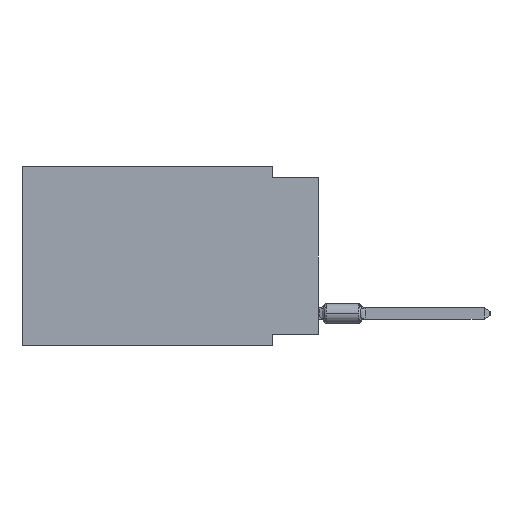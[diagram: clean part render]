
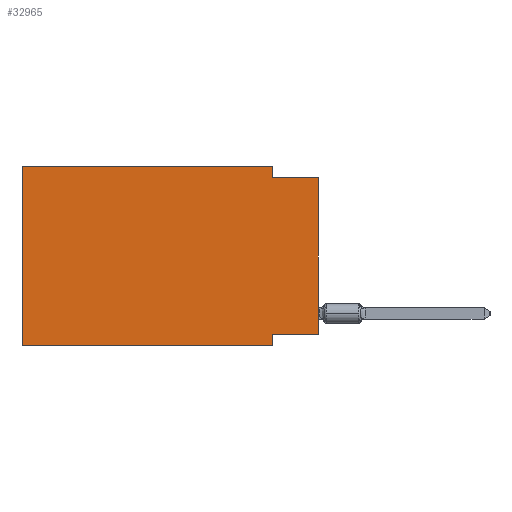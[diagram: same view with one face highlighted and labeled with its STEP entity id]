
A CAD part, left-side view. The second image highlights one B-rep face of the part: STEP entity #32965.
In plain terms, the highlighted planar face has unit normal (-1, 0, 0).
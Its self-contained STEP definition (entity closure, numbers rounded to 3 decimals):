
#2127 = CARTESIAN_POINT ( 'NONE',  ( 0., 2.54, -9.271 ) ) ;
#3897 = DIRECTION ( 'NONE',  ( 0., -1., 0. ) ) ;
#4107 = CARTESIAN_POINT ( 'NONE',  ( 0., 16.383, -9.906 ) ) ;
#6065 = ORIENTED_EDGE ( 'NONE', *, *, #28527, .F. ) ;
#7386 = DIRECTION ( 'NONE',  ( 0., 0., -1. ) ) ;
#9636 = ORIENTED_EDGE ( 'NONE', *, *, #46842, .T. ) ;
#9927 = ORIENTED_EDGE ( 'NONE', *, *, #17192, .F. ) ;
#12459 = LINE ( 'NONE', #16652, #61521 ) ;
#13066 = ORIENTED_EDGE ( 'NONE', *, *, #63137, .T. ) ;
#13706 = DIRECTION ( 'NONE',  ( 0., -1., 0. ) ) ;
#14728 = LINE ( 'NONE', #61482, #19033 ) ;
#15166 = CARTESIAN_POINT ( 'NONE',  ( 0., 2.54, -9.906 ) ) ;
#15357 = CARTESIAN_POINT ( 'NONE',  ( 0., 16.383, 0. ) ) ;
#16652 = CARTESIAN_POINT ( 'NONE',  ( 0., 16.383, 0. ) ) ;
#17192 = EDGE_CURVE ( 'NONE', #32666, #67689, #60074, .T. ) ;
#18453 = CARTESIAN_POINT ( 'NONE',  ( 0., 0., -9.271 ) ) ;
#19033 = VECTOR ( 'NONE', #13706, 1000. ) ;
#19069 = VECTOR ( 'NONE', #7386, 1000. ) ;
#20943 = FACE_OUTER_BOUND ( 'NONE', #68377, .T. ) ;
#20967 = VERTEX_POINT ( 'NONE', #50030 ) ;
#21779 = CARTESIAN_POINT ( 'NONE',  ( 0., 2.54, 0. ) ) ;
#24575 = ORIENTED_EDGE ( 'NONE', *, *, #39124, .F. ) ;
#25784 = EDGE_CURVE ( 'NONE', #51751, #32666, #12459, .T. ) ;
#25827 = PLANE ( 'NONE',  #32041 ) ;
#26291 = DIRECTION ( 'NONE',  ( 0., 0., 1. ) ) ;
#28527 = EDGE_CURVE ( 'NONE', #20967, #50083, #50545, .T. ) ;
#30525 = DIRECTION ( 'NONE',  ( 0., 0., -1. ) ) ;
#32041 = AXIS2_PLACEMENT_3D ( 'NONE', #15357, #63825, #53345 ) ;
#32348 = CARTESIAN_POINT ( 'NONE',  ( 0., 2.54, -0.635 ) ) ;
#32666 = VERTEX_POINT ( 'NONE', #46232 ) ;
#32965 = ADVANCED_FACE ( 'NONE', ( #20943 ), #25827, .F. ) ;
#33515 = ORIENTED_EDGE ( 'NONE', *, *, #57600, .F. ) ;
#34272 = VECTOR ( 'NONE', #26291, 1000. ) ;
#39124 = EDGE_CURVE ( 'NONE', #61178, #42774, #14728, .T. ) ;
#42774 = VERTEX_POINT ( 'NONE', #59467 ) ;
#43795 = VECTOR ( 'NONE', #44971, 1000. ) ;
#44689 = CARTESIAN_POINT ( 'NONE',  ( 0., 2.54, 0. ) ) ;
#44971 = DIRECTION ( 'NONE',  ( 0., 1., 0. ) ) ;
#46232 = CARTESIAN_POINT ( 'NONE',  ( 0., 16.383, 0. ) ) ;
#46842 = EDGE_CURVE ( 'NONE', #51751, #48183, #62115, .T. ) ;
#47285 = VECTOR ( 'NONE', #3897, 1000. ) ;
#48183 = VERTEX_POINT ( 'NONE', #58278 ) ;
#48239 = CARTESIAN_POINT ( 'NONE',  ( 0., 16.383, 0. ) ) ;
#49488 = ORIENTED_EDGE ( 'NONE', *, *, #25784, .F. ) ;
#50030 = CARTESIAN_POINT ( 'NONE',  ( 0., 0., -9.271 ) ) ;
#50083 = VERTEX_POINT ( 'NONE', #2127 ) ;
#50545 = LINE ( 'NONE', #18453, #43795 ) ;
#51751 = VERTEX_POINT ( 'NONE', #4107 ) ;
#53345 = DIRECTION ( 'NONE',  ( 0., 0., -1. ) ) ;
#54844 = DIRECTION ( 'NONE',  ( 0., -1., 0. ) ) ;
#55005 = DIRECTION ( 'NONE',  ( 0., 0., 1. ) ) ;
#56180 = VECTOR ( 'NONE', #30525, 1000. ) ;
#57600 = EDGE_CURVE ( 'NONE', #67689, #61178, #61053, .T. ) ;
#58278 = CARTESIAN_POINT ( 'NONE',  ( 0., 2.54, -9.906 ) ) ;
#58937 = VECTOR ( 'NONE', #54844, 1000. ) ;
#59467 = CARTESIAN_POINT ( 'NONE',  ( 0., 0., -0.635 ) ) ;
#60074 = LINE ( 'NONE', #48239, #58937 ) ;
#60709 = EDGE_CURVE ( 'NONE', #50083, #48183, #62254, .T. ) ;
#61053 = LINE ( 'NONE', #44689, #19069 ) ;
#61178 = VERTEX_POINT ( 'NONE', #32348 ) ;
#61482 = CARTESIAN_POINT ( 'NONE',  ( 0., 0., -0.635 ) ) ;
#61521 = VECTOR ( 'NONE', #55005, 1000. ) ;
#62115 = LINE ( 'NONE', #66692, #47285 ) ;
#62254 = LINE ( 'NONE', #15166, #56180 ) ;
#63137 = EDGE_CURVE ( 'NONE', #20967, #42774, #68498, .T. ) ;
#63255 = CARTESIAN_POINT ( 'NONE',  ( 0., 0., 0. ) ) ;
#63825 = DIRECTION ( 'NONE',  ( 1., 0., 0. ) ) ;
#65835 = ORIENTED_EDGE ( 'NONE', *, *, #60709, .F. ) ;
#66692 = CARTESIAN_POINT ( 'NONE',  ( 0., 16.383, -9.906 ) ) ;
#67689 = VERTEX_POINT ( 'NONE', #21779 ) ;
#68377 = EDGE_LOOP ( 'NONE', ( #13066, #24575, #33515, #9927, #49488, #9636, #65835, #6065 ) ) ;
#68498 = LINE ( 'NONE', #63255, #34272 ) ;
